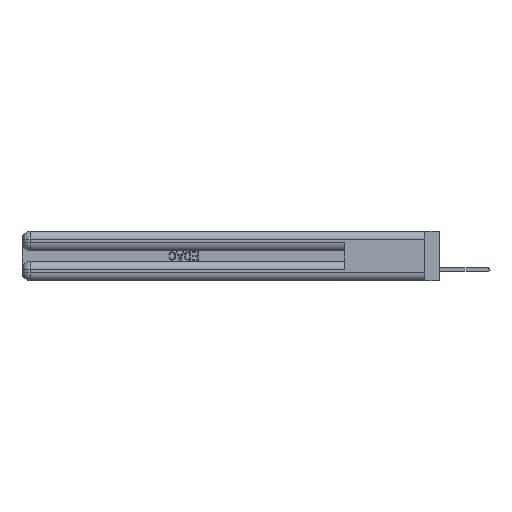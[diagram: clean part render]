
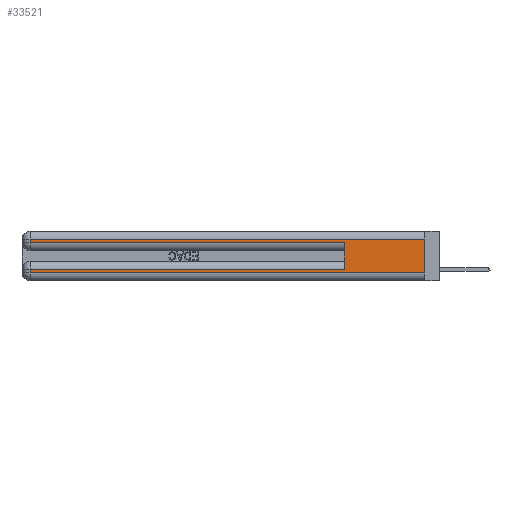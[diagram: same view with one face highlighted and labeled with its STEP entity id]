
A CAD part, left-side view. The second image highlights one B-rep face of the part: STEP entity #33521.
In plain terms, the highlighted planar face has unit normal (-1, 0, 0).
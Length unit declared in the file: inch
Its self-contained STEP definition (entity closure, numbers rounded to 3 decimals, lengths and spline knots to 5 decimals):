
#1610 = EDGE_CURVE ( 'NONE', #27800, #24452, #10909, .T. ) ;
#4247 = CARTESIAN_POINT ( 'NONE',  ( 0., 2.94, 0.31 ) ) ;
#4762 = FACE_OUTER_BOUND ( 'NONE', #10866, .T. ) ;
#6252 = EDGE_CURVE ( 'NONE', #9104, #46776, #6489, .T. ) ;
#6489 = LINE ( 'NONE', #8673, #43284 ) ;
#6576 = VECTOR ( 'NONE', #44567, 39.37008 ) ;
#6613 = ORIENTED_EDGE ( 'NONE', *, *, #16390, .T. ) ;
#7250 = CARTESIAN_POINT ( 'NONE',  ( 0., 0., 0.31 ) ) ;
#7423 = ORIENTED_EDGE ( 'NONE', *, *, #18877, .F. ) ;
#8135 = CARTESIAN_POINT ( 'NONE',  ( 0., 0., 0.285 ) ) ;
#8673 = CARTESIAN_POINT ( 'NONE',  ( 0., 0., 0.06 ) ) ;
#8995 = CARTESIAN_POINT ( 'NONE',  ( 0., 0.6, 0.285 ) ) ;
#9104 = VERTEX_POINT ( 'NONE', #36612 ) ;
#9763 = EDGE_CURVE ( 'NONE', #18081, #16218, #37594, .T. ) ;
#10545 = ORIENTED_EDGE ( 'NONE', *, *, #46182, .T. ) ;
#10866 = EDGE_LOOP ( 'NONE', ( #7423, #36143, #38355, #10545, #24681, #24726, #6613, #46271 ) ) ;
#10909 = LINE ( 'NONE', #30857, #24095 ) ;
#11372 = DIRECTION ( 'NONE',  ( 0., 1., 0. ) ) ;
#13036 = LINE ( 'NONE', #36731, #41377 ) ;
#13136 = CARTESIAN_POINT ( 'NONE',  ( 0., 0.6, 0.085 ) ) ;
#14804 = EDGE_CURVE ( 'NONE', #24452, #45260, #31241, .T. ) ;
#15228 = CARTESIAN_POINT ( 'NONE',  ( 0., 2.94, 0.37 ) ) ;
#16218 = VERTEX_POINT ( 'NONE', #8995 ) ;
#16390 = EDGE_CURVE ( 'NONE', #36290, #9104, #13036, .T. ) ;
#18081 = VERTEX_POINT ( 'NONE', #13136 ) ;
#18122 = CARTESIAN_POINT ( 'NONE',  ( 0., 2.94, 0.285 ) ) ;
#18877 = EDGE_CURVE ( 'NONE', #27800, #46776, #30899, .T. ) ;
#23063 = DIRECTION ( 'NONE',  ( 0., 0., -1. ) ) ;
#23319 = AXIS2_PLACEMENT_3D ( 'NONE', #48432, #29201, #25724 ) ;
#24095 = VECTOR ( 'NONE', #11372, 39.37008 ) ;
#24236 = DIRECTION ( 'NONE',  ( 0., 0., 1. ) ) ;
#24292 = VECTOR ( 'NONE', #23063, 39.37008 ) ;
#24406 = CARTESIAN_POINT ( 'NONE',  ( 0., 0.6, 0.145 ) ) ;
#24452 = VERTEX_POINT ( 'NONE', #4247 ) ;
#24681 = ORIENTED_EDGE ( 'NONE', *, *, #9763, .F. ) ;
#24726 = ORIENTED_EDGE ( 'NONE', *, *, #40772, .T. ) ;
#25724 = DIRECTION ( 'NONE',  ( 0., 0., -1. ) ) ;
#26053 = CARTESIAN_POINT ( 'NONE',  ( 0., 0., 0.085 ) ) ;
#26163 = VECTOR ( 'NONE', #24236, 39.37008 ) ;
#26538 = LINE ( 'NONE', #26053, #6576 ) ;
#27800 = VERTEX_POINT ( 'NONE', #7250 ) ;
#28878 = DIRECTION ( 'NONE',  ( 0., 0., -1. ) ) ;
#29201 = DIRECTION ( 'NONE',  ( 1., 0., 0. ) ) ;
#30857 = CARTESIAN_POINT ( 'NONE',  ( 0., 0., 0.31 ) ) ;
#30899 = LINE ( 'NONE', #34773, #24292 ) ;
#30989 = CARTESIAN_POINT ( 'NONE',  ( 0., 0., 0.06 ) ) ;
#31241 = LINE ( 'NONE', #15228, #44540 ) ;
#33521 = ADVANCED_FACE ( 'NONE', ( #4762 ), #44744, .F. ) ;
#34773 = CARTESIAN_POINT ( 'NONE',  ( 0., 0., 0.37 ) ) ;
#36143 = ORIENTED_EDGE ( 'NONE', *, *, #1610, .T. ) ;
#36290 = VERTEX_POINT ( 'NONE', #48955 ) ;
#36612 = CARTESIAN_POINT ( 'NONE',  ( 0., 2.94, 0.06 ) ) ;
#36731 = CARTESIAN_POINT ( 'NONE',  ( 0., 2.94, 0.37 ) ) ;
#37073 = DIRECTION ( 'NONE',  ( 0., 0., -1. ) ) ;
#37594 = LINE ( 'NONE', #24406, #26163 ) ;
#38355 = ORIENTED_EDGE ( 'NONE', *, *, #14804, .T. ) ;
#38655 = LINE ( 'NONE', #8135, #44066 ) ;
#38942 = DIRECTION ( 'NONE',  ( 0., -1., 0. ) ) ;
#40772 = EDGE_CURVE ( 'NONE', #18081, #36290, #26538, .T. ) ;
#41377 = VECTOR ( 'NONE', #37073, 39.37008 ) ;
#43284 = VECTOR ( 'NONE', #49478, 39.37008 ) ;
#44066 = VECTOR ( 'NONE', #38942, 39.37008 ) ;
#44540 = VECTOR ( 'NONE', #28878, 39.37008 ) ;
#44567 = DIRECTION ( 'NONE',  ( 0., 1., 0. ) ) ;
#44744 = PLANE ( 'NONE',  #23319 ) ;
#45260 = VERTEX_POINT ( 'NONE', #18122 ) ;
#46182 = EDGE_CURVE ( 'NONE', #45260, #16218, #38655, .T. ) ;
#46271 = ORIENTED_EDGE ( 'NONE', *, *, #6252, .T. ) ;
#46776 = VERTEX_POINT ( 'NONE', #30989 ) ;
#48432 = CARTESIAN_POINT ( 'NONE',  ( 0., 0., 0.37 ) ) ;
#48955 = CARTESIAN_POINT ( 'NONE',  ( 0., 2.94, 0.085 ) ) ;
#49478 = DIRECTION ( 'NONE',  ( 0., -1., 0. ) ) ;
